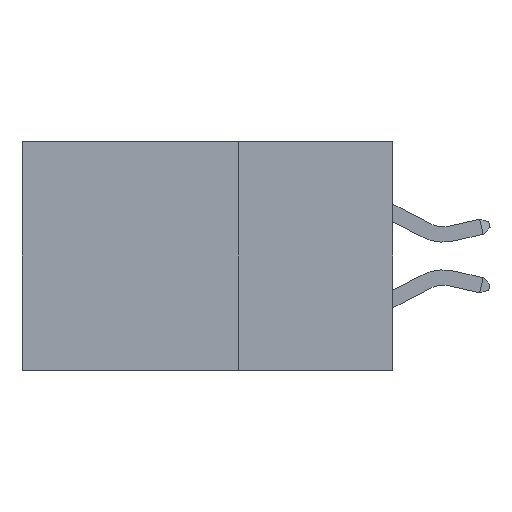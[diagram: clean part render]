
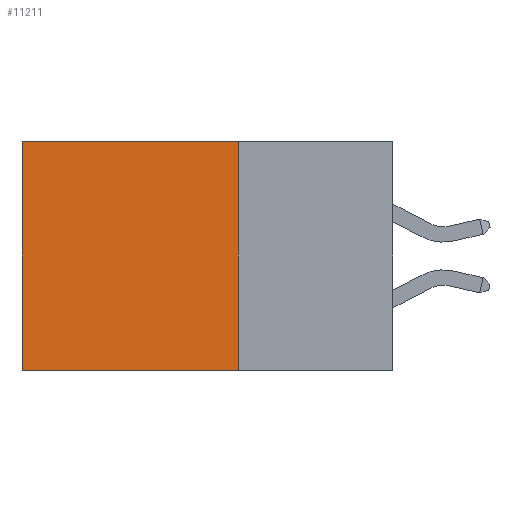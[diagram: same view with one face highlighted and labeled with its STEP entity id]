
A CAD part, left-side view. The second image highlights one B-rep face of the part: STEP entity #11211.
In plain terms, the highlighted planar face has unit normal (-1, 0, 0).
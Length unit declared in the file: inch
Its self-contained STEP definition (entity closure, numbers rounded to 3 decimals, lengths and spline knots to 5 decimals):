
#225 = CARTESIAN_POINT ( 'NONE',  ( 0.2875, 0.6, 0. ) ) ;
#1168 = ORIENTED_EDGE ( 'NONE', *, *, #8937, .T. ) ;
#1230 = EDGE_CURVE ( 'NONE', #9238, #10030, #10430, .T. ) ;
#2149 = CARTESIAN_POINT ( 'NONE',  ( 0.2875, 0.25, -0.37 ) ) ;
#2446 = CARTESIAN_POINT ( 'NONE',  ( 0.2875, 0.25, 0. ) ) ;
#2701 = VECTOR ( 'NONE', #6788, 39.37008 ) ;
#2831 = FACE_OUTER_BOUND ( 'NONE', #3681, .T. ) ;
#2913 = EDGE_CURVE ( 'NONE', #19381, #9238, #9915, .T. ) ;
#3674 = CARTESIAN_POINT ( 'NONE',  ( 0.2875, 0.6, 0. ) ) ;
#3681 = EDGE_LOOP ( 'NONE', ( #14337, #15559, #15705, #1168 ) ) ;
#3792 = LINE ( 'NONE', #16415, #5542 ) ;
#4069 = CARTESIAN_POINT ( 'NONE',  ( 0.2875, 0.25, -0.37 ) ) ;
#5542 = VECTOR ( 'NONE', #19446, 39.37008 ) ;
#5753 = DIRECTION ( 'NONE',  ( 0., 0., -1. ) ) ;
#5964 = DIRECTION ( 'NONE',  ( 1., 0., 0. ) ) ;
#6788 = DIRECTION ( 'NONE',  ( 0., 0., -1. ) ) ;
#7368 = CARTESIAN_POINT ( 'NONE',  ( 0.2875, 0.25, 0. ) ) ;
#8937 = EDGE_CURVE ( 'NONE', #19381, #18803, #3792, .T. ) ;
#9238 = VERTEX_POINT ( 'NONE', #2149 ) ;
#9915 = LINE ( 'NONE', #2446, #14147 ) ;
#10030 = VERTEX_POINT ( 'NONE', #11467 ) ;
#10409 = EDGE_CURVE ( 'NONE', #18803, #10030, #17499, .T. ) ;
#10430 = LINE ( 'NONE', #4069, #16780 ) ;
#11211 = ADVANCED_FACE ( 'NONE', ( #2831 ), #13441, .F. ) ;
#11383 = AXIS2_PLACEMENT_3D ( 'NONE', #7368, #5964, #5753 ) ;
#11467 = CARTESIAN_POINT ( 'NONE',  ( 0.2875, 0.6, -0.37 ) ) ;
#11942 = DIRECTION ( 'NONE',  ( 0., 1., 0. ) ) ;
#13050 = DIRECTION ( 'NONE',  ( 0., 0., -1. ) ) ;
#13441 = PLANE ( 'NONE',  #11383 ) ;
#14147 = VECTOR ( 'NONE', #13050, 39.37008 ) ;
#14337 = ORIENTED_EDGE ( 'NONE', *, *, #10409, .T. ) ;
#15559 = ORIENTED_EDGE ( 'NONE', *, *, #1230, .F. ) ;
#15705 = ORIENTED_EDGE ( 'NONE', *, *, #2913, .F. ) ;
#16415 = CARTESIAN_POINT ( 'NONE',  ( 0.2875, 0.25, 0. ) ) ;
#16780 = VECTOR ( 'NONE', #11942, 39.37008 ) ;
#17499 = LINE ( 'NONE', #3674, #2701 ) ;
#18803 = VERTEX_POINT ( 'NONE', #225 ) ;
#18889 = CARTESIAN_POINT ( 'NONE',  ( 0.2875, 0.25, 0. ) ) ;
#19381 = VERTEX_POINT ( 'NONE', #18889 ) ;
#19446 = DIRECTION ( 'NONE',  ( 0., 1., 0. ) ) ;
